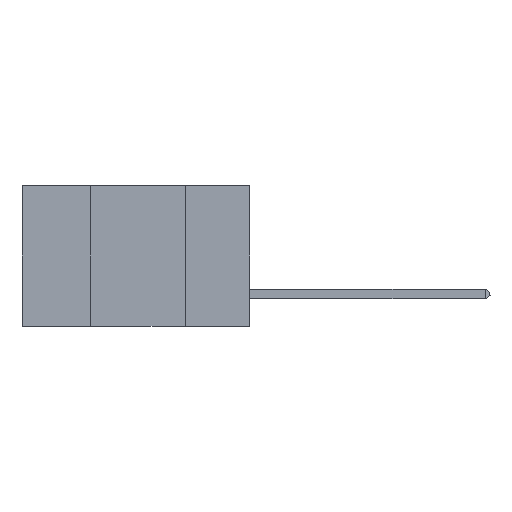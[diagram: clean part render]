
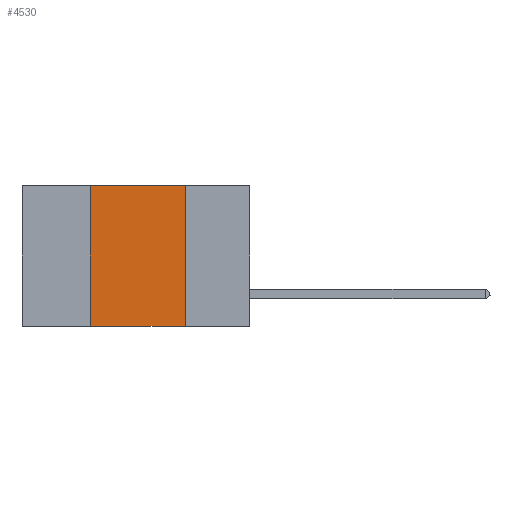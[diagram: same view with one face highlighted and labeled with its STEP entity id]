
A CAD part, left-side view. The second image highlights one B-rep face of the part: STEP entity #4530.
In plain terms, the highlighted planar face has unit normal (-1, 0, 0).
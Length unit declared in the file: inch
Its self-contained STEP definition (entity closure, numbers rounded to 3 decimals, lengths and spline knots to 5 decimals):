
#366 = VECTOR ( 'NONE', #12999, 39.37008 ) ;
#379 = VERTEX_POINT ( 'NONE', #15606 ) ;
#605 = VERTEX_POINT ( 'NONE', #9609 ) ;
#1081 = DIRECTION ( 'NONE',  ( 0., -1., 0. ) ) ;
#2394 = CARTESIAN_POINT ( 'NONE',  ( 0., 0.6, -0.37 ) ) ;
#4192 = EDGE_CURVE ( 'NONE', #379, #13089, #11621, .T. ) ;
#4259 = VERTEX_POINT ( 'NONE', #8281 ) ;
#4527 = EDGE_CURVE ( 'NONE', #4259, #379, #5103, .T. ) ;
#4530 = ADVANCED_FACE ( 'NONE', ( #11697 ), #16876, .F. ) ;
#5027 = LINE ( 'NONE', #2394, #15047 ) ;
#5103 = LINE ( 'NONE', #13177, #366 ) ;
#6119 = EDGE_LOOP ( 'NONE', ( #10503, #9140, #11074, #15684 ) ) ;
#6428 = DIRECTION ( 'NONE',  ( 0., -1., 0. ) ) ;
#7387 = CARTESIAN_POINT ( 'NONE',  ( 0., 0.17, 0. ) ) ;
#7449 = VECTOR ( 'NONE', #1081, 39.37008 ) ;
#8281 = CARTESIAN_POINT ( 'NONE',  ( 0., 0.42, -0.37 ) ) ;
#9140 = ORIENTED_EDGE ( 'NONE', *, *, #4192, .F. ) ;
#9563 = EDGE_CURVE ( 'NONE', #13089, #605, #10023, .T. ) ;
#9609 = CARTESIAN_POINT ( 'NONE',  ( 0., 0.17, -0.37 ) ) ;
#10023 = LINE ( 'NONE', #7387, #15336 ) ;
#10503 = ORIENTED_EDGE ( 'NONE', *, *, #9563, .F. ) ;
#11074 = ORIENTED_EDGE ( 'NONE', *, *, #4527, .F. ) ;
#11524 = DIRECTION ( 'NONE',  ( 1., 0., 0. ) ) ;
#11621 = LINE ( 'NONE', #14524, #7449 ) ;
#11697 = FACE_OUTER_BOUND ( 'NONE', #6119, .T. ) ;
#11732 = CARTESIAN_POINT ( 'NONE',  ( 0., 0.17, 0. ) ) ;
#12999 = DIRECTION ( 'NONE',  ( 0., 0., 1. ) ) ;
#13089 = VERTEX_POINT ( 'NONE', #11732 ) ;
#13177 = CARTESIAN_POINT ( 'NONE',  ( 0., 0.42, 0. ) ) ;
#14328 = DIRECTION ( 'NONE',  ( 0., 0., -1. ) ) ;
#14524 = CARTESIAN_POINT ( 'NONE',  ( 0., 0.6, 0. ) ) ;
#15047 = VECTOR ( 'NONE', #6428, 39.37008 ) ;
#15336 = VECTOR ( 'NONE', #16782, 39.37008 ) ;
#15461 = AXIS2_PLACEMENT_3D ( 'NONE', #16957, #11524, #14328 ) ;
#15606 = CARTESIAN_POINT ( 'NONE',  ( 0., 0.42, 0. ) ) ;
#15684 = ORIENTED_EDGE ( 'NONE', *, *, #15743, .T. ) ;
#15743 = EDGE_CURVE ( 'NONE', #4259, #605, #5027, .T. ) ;
#16782 = DIRECTION ( 'NONE',  ( 0., 0., -1. ) ) ;
#16876 = PLANE ( 'NONE',  #15461 ) ;
#16957 = CARTESIAN_POINT ( 'NONE',  ( 0., 0.6, 0. ) ) ;
